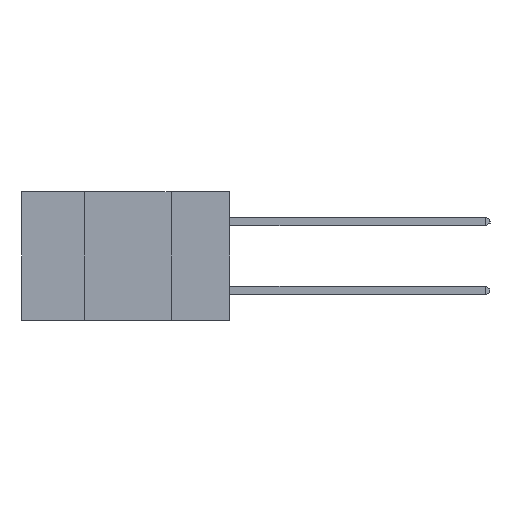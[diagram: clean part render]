
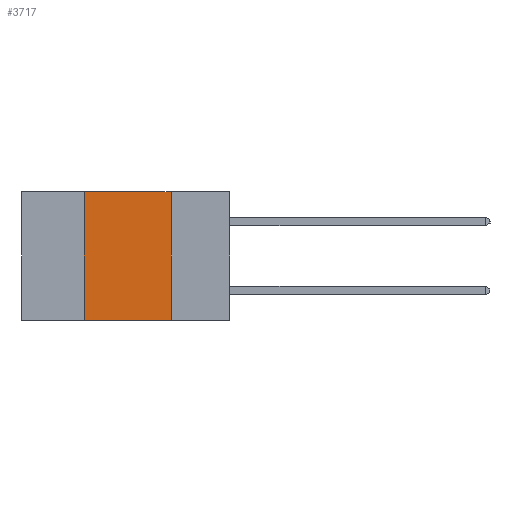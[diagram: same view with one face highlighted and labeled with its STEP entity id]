
A CAD part, left-side view. The second image highlights one B-rep face of the part: STEP entity #3717.
In plain terms, the highlighted planar face has unit normal (-1, 0, 0).
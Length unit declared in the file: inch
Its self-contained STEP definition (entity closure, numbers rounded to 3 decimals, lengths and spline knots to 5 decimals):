
#635 = CARTESIAN_POINT ( 'NONE',  ( 0., 0.6, 0. ) ) ;
#1269 = LINE ( 'NONE', #23407, #2495 ) ;
#2495 = VECTOR ( 'NONE', #15566, 39.37008 ) ;
#2885 = DIRECTION ( 'NONE',  ( 0., 0., -1. ) ) ;
#3334 = DIRECTION ( 'NONE',  ( 0., -1., 0. ) ) ;
#3717 = ADVANCED_FACE ( 'NONE', ( #4538 ), #31414, .F. ) ;
#3952 = VECTOR ( 'NONE', #3334, 39.37008 ) ;
#4268 = CARTESIAN_POINT ( 'NONE',  ( 0., 0.17, -0.37 ) ) ;
#4538 = FACE_OUTER_BOUND ( 'NONE', #14012, .T. ) ;
#4611 = CARTESIAN_POINT ( 'NONE',  ( 0., 0.6, 0. ) ) ;
#4873 = AXIS2_PLACEMENT_3D ( 'NONE', #4611, #15619, #34040 ) ;
#6222 = DIRECTION ( 'NONE',  ( 0., 0., 1. ) ) ;
#6371 = VECTOR ( 'NONE', #6222, 39.37008 ) ;
#6745 = CARTESIAN_POINT ( 'NONE',  ( 0., 0.17, 0. ) ) ;
#11111 = LINE ( 'NONE', #635, #3952 ) ;
#11757 = ORIENTED_EDGE ( 'NONE', *, *, #24769, .F. ) ;
#14012 = EDGE_LOOP ( 'NONE', ( #17124, #31969, #11757, #19638 ) ) ;
#15566 = DIRECTION ( 'NONE',  ( 0., -1., 0. ) ) ;
#15619 = DIRECTION ( 'NONE',  ( 1., 0., 0. ) ) ;
#16849 = CARTESIAN_POINT ( 'NONE',  ( 0., 0.42, 0. ) ) ;
#17124 = ORIENTED_EDGE ( 'NONE', *, *, #17634, .F. ) ;
#17279 = VERTEX_POINT ( 'NONE', #6745 ) ;
#17634 = EDGE_CURVE ( 'NONE', #17279, #30885, #33153, .T. ) ;
#18781 = CARTESIAN_POINT ( 'NONE',  ( 0., 0.42, -0.37 ) ) ;
#19638 = ORIENTED_EDGE ( 'NONE', *, *, #28955, .T. ) ;
#20641 = VERTEX_POINT ( 'NONE', #33574 ) ;
#21523 = CARTESIAN_POINT ( 'NONE',  ( 0., 0.17, 0. ) ) ;
#23407 = CARTESIAN_POINT ( 'NONE',  ( 0., 0.6, -0.37 ) ) ;
#24769 = EDGE_CURVE ( 'NONE', #25203, #20641, #27602, .T. ) ;
#25203 = VERTEX_POINT ( 'NONE', #18781 ) ;
#25390 = VECTOR ( 'NONE', #2885, 39.37008 ) ;
#26024 = EDGE_CURVE ( 'NONE', #20641, #17279, #11111, .T. ) ;
#27602 = LINE ( 'NONE', #16849, #6371 ) ;
#28955 = EDGE_CURVE ( 'NONE', #25203, #30885, #1269, .T. ) ;
#30885 = VERTEX_POINT ( 'NONE', #4268 ) ;
#31414 = PLANE ( 'NONE',  #4873 ) ;
#31969 = ORIENTED_EDGE ( 'NONE', *, *, #26024, .F. ) ;
#33153 = LINE ( 'NONE', #21523, #25390 ) ;
#33574 = CARTESIAN_POINT ( 'NONE',  ( 0., 0.42, 0. ) ) ;
#34040 = DIRECTION ( 'NONE',  ( 0., 0., -1. ) ) ;
